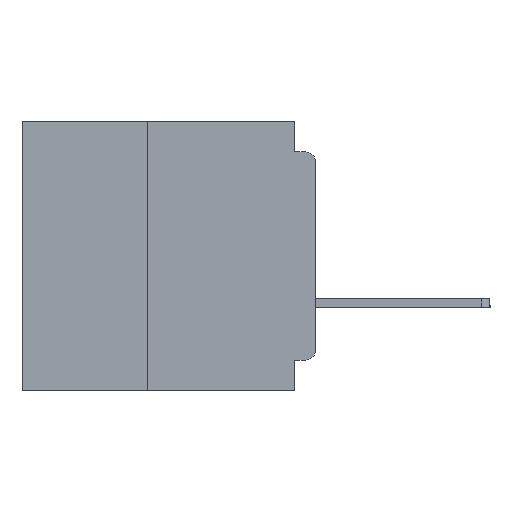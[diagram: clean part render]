
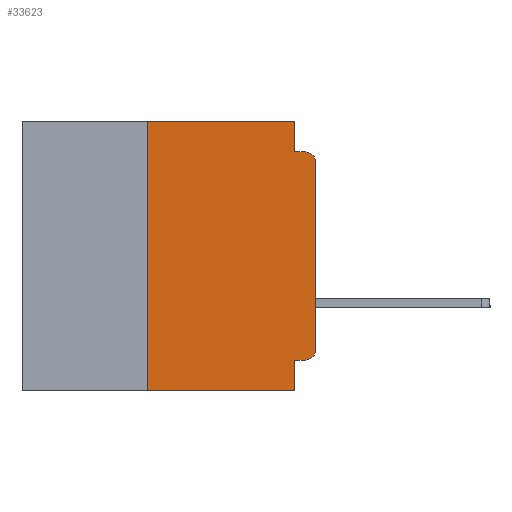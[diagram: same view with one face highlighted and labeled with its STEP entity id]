
A CAD part, left-side view. The second image highlights one B-rep face of the part: STEP entity #33623.
In plain terms, the highlighted planar face has unit normal (-1, 0, 0).
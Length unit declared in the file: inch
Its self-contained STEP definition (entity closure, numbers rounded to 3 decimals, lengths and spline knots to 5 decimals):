
#3 = CARTESIAN_POINT ( 'NONE',  ( 0., 0., -0.045 ) ) ;
#860 = CARTESIAN_POINT ( 'NONE',  ( 0., 0.031, -0.355 ) ) ;
#1571 = DIRECTION ( 'NONE',  ( 0., 0., -1. ) ) ;
#1653 = CARTESIAN_POINT ( 'NONE',  ( 0., 0., -0.06 ) ) ;
#2112 = CARTESIAN_POINT ( 'NONE',  ( 0., 0.015, -0.355 ) ) ;
#2900 = EDGE_CURVE ( 'NONE', #20306, #45564, #27234, .T. ) ;
#3197 = ORIENTED_EDGE ( 'NONE', *, *, #17780, .F. ) ;
#4483 = ORIENTED_EDGE ( 'NONE', *, *, #6186, .T. ) ;
#5075 = CIRCLE ( 'NONE', #8962, 0.015 ) ;
#5140 = CARTESIAN_POINT ( 'NONE',  ( 0., 0.031, -0.4 ) ) ;
#6018 = CARTESIAN_POINT ( 'NONE',  ( 0., 0., 0. ) ) ;
#6186 = EDGE_CURVE ( 'NONE', #34339, #16452, #39124, .T. ) ;
#6233 = DIRECTION ( 'NONE',  ( 0., 0., -1. ) ) ;
#7089 = VECTOR ( 'NONE', #31333, 39.37008 ) ;
#7336 = VECTOR ( 'NONE', #27371, 39.37008 ) ;
#7454 = DIRECTION ( 'NONE',  ( 0., 1., 0. ) ) ;
#7460 = VERTEX_POINT ( 'NONE', #1653 ) ;
#8320 = ORIENTED_EDGE ( 'NONE', *, *, #28168, .F. ) ;
#8962 = AXIS2_PLACEMENT_3D ( 'NONE', #40041, #18982, #43558 ) ;
#9594 = DIRECTION ( 'NONE',  ( 0., 0., 1. ) ) ;
#9808 = EDGE_CURVE ( 'NONE', #16452, #7460, #18578, .T. ) ;
#10762 = LINE ( 'NONE', #20713, #20130 ) ;
#11365 = ORIENTED_EDGE ( 'NONE', *, *, #13314, .F. ) ;
#11967 = AXIS2_PLACEMENT_3D ( 'NONE', #19247, #22782, #1571 ) ;
#12463 = EDGE_CURVE ( 'NONE', #7460, #26769, #5075, .T. ) ;
#13314 = EDGE_CURVE ( 'NONE', #42363, #33637, #33222, .T. ) ;
#13514 = ORIENTED_EDGE ( 'NONE', *, *, #14541, .F. ) ;
#14541 = EDGE_CURVE ( 'NONE', #33458, #20306, #35255, .T. ) ;
#14665 = FACE_OUTER_BOUND ( 'NONE', #25340, .T. ) ;
#15656 = EDGE_CURVE ( 'NONE', #22464, #33637, #10762, .T. ) ;
#15662 = PLANE ( 'NONE',  #11967 ) ;
#16452 = VERTEX_POINT ( 'NONE', #45441 ) ;
#16681 = VECTOR ( 'NONE', #35234, 39.37008 ) ;
#17780 = EDGE_CURVE ( 'NONE', #45564, #26769, #37092, .T. ) ;
#18175 = CARTESIAN_POINT ( 'NONE',  ( 0., 0.25, 0. ) ) ;
#18578 = LINE ( 'NONE', #6018, #25300 ) ;
#18582 = ORIENTED_EDGE ( 'NONE', *, *, #15656, .T. ) ;
#18982 = DIRECTION ( 'NONE',  ( -1., 0., 0. ) ) ;
#19247 = CARTESIAN_POINT ( 'NONE',  ( 0., 0.437, 0. ) ) ;
#19306 = LINE ( 'NONE', #32176, #20381 ) ;
#20130 = VECTOR ( 'NONE', #45294, 39.37008 ) ;
#20306 = VERTEX_POINT ( 'NONE', #42811 ) ;
#20381 = VECTOR ( 'NONE', #7454, 39.37008 ) ;
#20713 = CARTESIAN_POINT ( 'NONE',  ( 0., 0.437, -0.4 ) ) ;
#21014 = AXIS2_PLACEMENT_3D ( 'NONE', #29511, #29426, #29379 ) ;
#22464 = VERTEX_POINT ( 'NONE', #28881 ) ;
#22782 = DIRECTION ( 'NONE',  ( 1., 0., 0. ) ) ;
#23081 = ORIENTED_EDGE ( 'NONE', *, *, #32274, .F. ) ;
#23804 = CARTESIAN_POINT ( 'NONE',  ( 0., 0.25, -0.4 ) ) ;
#23868 = CARTESIAN_POINT ( 'NONE',  ( 0., 0.031, -0.4 ) ) ;
#24804 = DIRECTION ( 'NONE',  ( 0., -1., 0. ) ) ;
#25300 = VECTOR ( 'NONE', #9594, 39.37008 ) ;
#25340 = EDGE_LOOP ( 'NONE', ( #29639, #26977, #3197, #28131, #13514, #23081, #18582, #11365, #8320, #4483 ) ) ;
#26158 = LINE ( 'NONE', #23804, #7336 ) ;
#26769 = VERTEX_POINT ( 'NONE', #33221 ) ;
#26977 = ORIENTED_EDGE ( 'NONE', *, *, #12463, .T. ) ;
#27234 = LINE ( 'NONE', #41186, #16681 ) ;
#27371 = DIRECTION ( 'NONE',  ( 0., 0., 1. ) ) ;
#27789 = CARTESIAN_POINT ( 'NONE',  ( 0., 0.437, 0. ) ) ;
#28131 = ORIENTED_EDGE ( 'NONE', *, *, #2900, .F. ) ;
#28168 = EDGE_CURVE ( 'NONE', #34339, #42363, #19306, .T. ) ;
#28881 = CARTESIAN_POINT ( 'NONE',  ( 0., 0.25, -0.4 ) ) ;
#29379 = DIRECTION ( 'NONE',  ( 0., 0., -1. ) ) ;
#29426 = DIRECTION ( 'NONE',  ( -1., 0., 0. ) ) ;
#29511 = CARTESIAN_POINT ( 'NONE',  ( 0., 0.015, -0.34 ) ) ;
#29639 = ORIENTED_EDGE ( 'NONE', *, *, #9808, .T. ) ;
#31333 = DIRECTION ( 'NONE',  ( 0., -1., 0. ) ) ;
#32176 = CARTESIAN_POINT ( 'NONE',  ( 0., 0., -0.355 ) ) ;
#32274 = EDGE_CURVE ( 'NONE', #22464, #33458, #26158, .T. ) ;
#33221 = CARTESIAN_POINT ( 'NONE',  ( 0., 0.015, -0.045 ) ) ;
#33222 = LINE ( 'NONE', #23868, #34289 ) ;
#33458 = VERTEX_POINT ( 'NONE', #18175 ) ;
#33623 = ADVANCED_FACE ( 'NONE', ( #14665 ), #15662, .F. ) ;
#33637 = VERTEX_POINT ( 'NONE', #5140 ) ;
#34289 = VECTOR ( 'NONE', #6233, 39.37008 ) ;
#34339 = VERTEX_POINT ( 'NONE', #2112 ) ;
#35234 = DIRECTION ( 'NONE',  ( 0., 0., -1. ) ) ;
#35255 = LINE ( 'NONE', #27789, #7089 ) ;
#37092 = LINE ( 'NONE', #3, #38152 ) ;
#38152 = VECTOR ( 'NONE', #24804, 39.37008 ) ;
#39124 = CIRCLE ( 'NONE', #21014, 0.015 ) ;
#39629 = CARTESIAN_POINT ( 'NONE',  ( 0., 0.031, -0.045 ) ) ;
#40041 = CARTESIAN_POINT ( 'NONE',  ( 0., 0.015, -0.06 ) ) ;
#41186 = CARTESIAN_POINT ( 'NONE',  ( 0., 0.031, 0. ) ) ;
#42363 = VERTEX_POINT ( 'NONE', #860 ) ;
#42811 = CARTESIAN_POINT ( 'NONE',  ( 0., 0.031, 0. ) ) ;
#43558 = DIRECTION ( 'NONE',  ( 0., 0., -1. ) ) ;
#45294 = DIRECTION ( 'NONE',  ( 0., -1., 0. ) ) ;
#45441 = CARTESIAN_POINT ( 'NONE',  ( 0., 0., -0.34 ) ) ;
#45564 = VERTEX_POINT ( 'NONE', #39629 ) ;
